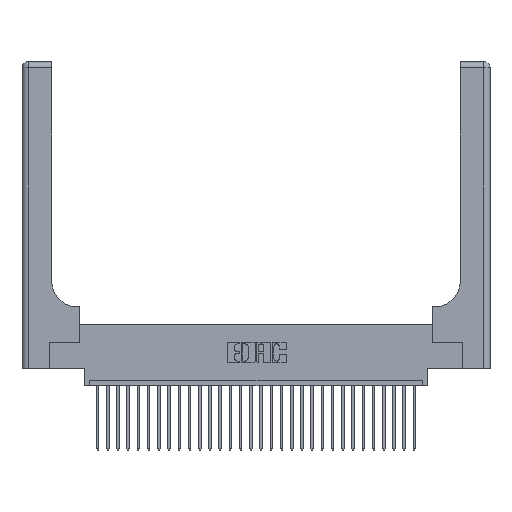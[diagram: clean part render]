
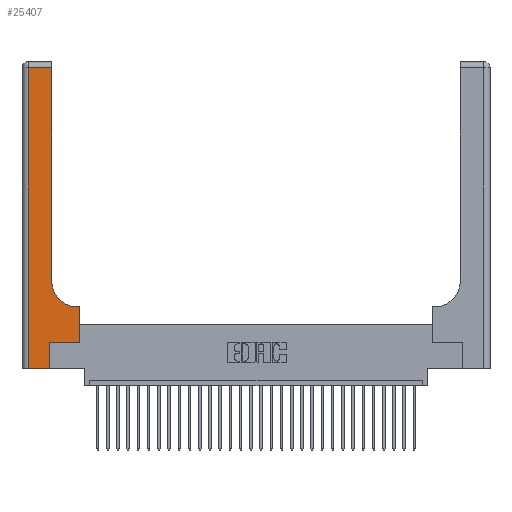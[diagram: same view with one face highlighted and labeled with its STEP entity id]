
A CAD part, top view. The second image highlights one B-rep face of the part: STEP entity #25407.
In plain terms, the highlighted planar face has unit normal (0, 0, 1).
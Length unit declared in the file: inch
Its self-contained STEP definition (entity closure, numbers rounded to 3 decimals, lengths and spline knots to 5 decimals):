
#1263 = CARTESIAN_POINT ( 'NONE',  ( 0.5415, 0.85, 0.37 ) ) ;
#1812 = FACE_OUTER_BOUND ( 'NONE', #27605, .T. ) ;
#2445 = CARTESIAN_POINT ( 'NONE',  ( 0.5415, 0.6, 0.37 ) ) ;
#2628 = EDGE_CURVE ( 'NONE', #19721, #12582, #14094, .T. ) ;
#2738 = CARTESIAN_POINT ( 'NONE',  ( 0.2915, 0.85, 0.37 ) ) ;
#2833 = VECTOR ( 'NONE', #13495, 39.37008 ) ;
#3415 = EDGE_CURVE ( 'NONE', #28434, #19721, #30053, .T. ) ;
#3424 = DIRECTION ( 'NONE',  ( 1., 0., 0. ) ) ;
#4033 = LINE ( 'NONE', #15360, #9617 ) ;
#4119 = EDGE_CURVE ( 'NONE', #24742, #16870, #18532, .T. ) ;
#4542 = VECTOR ( 'NONE', #12631, 39.37008 ) ;
#4820 = VECTOR ( 'NONE', #21781, 39.37008 ) ;
#4957 = LINE ( 'NONE', #10661, #13817 ) ;
#4981 = DIRECTION ( 'NONE',  ( 0., 0., -1. ) ) ;
#6355 = CARTESIAN_POINT ( 'NONE',  ( 0.5585, 0.25, 0.37 ) ) ;
#7140 = EDGE_CURVE ( 'NONE', #30685, #24742, #9123, .T. ) ;
#7196 = AXIS2_PLACEMENT_3D ( 'NONE', #23761, #4981, #26261 ) ;
#7293 = ORIENTED_EDGE ( 'NONE', *, *, #10783, .T. ) ;
#7933 = CARTESIAN_POINT ( 'NONE',  ( 0.5585, 0.25, 0.37 ) ) ;
#9074 = CARTESIAN_POINT ( 'NONE',  ( 0.269, 0.25, 0.37 ) ) ;
#9123 = LINE ( 'NONE', #6355, #10249 ) ;
#9617 = VECTOR ( 'NONE', #3424, 39.37008 ) ;
#10152 = ORIENTED_EDGE ( 'NONE', *, *, #29019, .T. ) ;
#10249 = VECTOR ( 'NONE', #18937, 39.37008 ) ;
#10362 = CARTESIAN_POINT ( 'NONE',  ( 0.2915, 3., 0.37 ) ) ;
#10658 = CIRCLE ( 'NONE', #14907, 0.25 ) ;
#10661 = CARTESIAN_POINT ( 'NONE',  ( 0., 2.94, 0.37 ) ) ;
#10696 = CARTESIAN_POINT ( 'NONE',  ( 0.06, 2.94, 0.37 ) ) ;
#10783 = EDGE_CURVE ( 'NONE', #23020, #30685, #4033, .T. ) ;
#10990 = DIRECTION ( 'NONE',  ( 0., 0., -1. ) ) ;
#11312 = ORIENTED_EDGE ( 'NONE', *, *, #7140, .T. ) ;
#11572 = DIRECTION ( 'NONE',  ( 1., 0., 0. ) ) ;
#12044 = EDGE_CURVE ( 'NONE', #16870, #23280, #10658, .T. ) ;
#12126 = ORIENTED_EDGE ( 'NONE', *, *, #29683, .T. ) ;
#12237 = PLANE ( 'NONE',  #7196 ) ;
#12582 = VERTEX_POINT ( 'NONE', #22857 ) ;
#12631 = DIRECTION ( 'NONE',  ( 0., 1., 0. ) ) ;
#12977 = ORIENTED_EDGE ( 'NONE', *, *, #2628, .T. ) ;
#13495 = DIRECTION ( 'NONE',  ( 0., 1., 0. ) ) ;
#13817 = VECTOR ( 'NONE', #27359, 39.37008 ) ;
#14094 = LINE ( 'NONE', #14251, #29005 ) ;
#14251 = CARTESIAN_POINT ( 'NONE',  ( 0., 0., 0.37 ) ) ;
#14380 = CARTESIAN_POINT ( 'NONE',  ( 0.06, 3., 0.37 ) ) ;
#14668 = CARTESIAN_POINT ( 'NONE',  ( 0.2915, 0.6, 0.37 ) ) ;
#14854 = ORIENTED_EDGE ( 'NONE', *, *, #12044, .T. ) ;
#14907 = AXIS2_PLACEMENT_3D ( 'NONE', #1263, #10990, #27188 ) ;
#15360 = CARTESIAN_POINT ( 'NONE',  ( 0.269, 0.25, 0.37 ) ) ;
#15441 = EDGE_CURVE ( 'NONE', #23280, #19581, #30542, .T. ) ;
#16237 = CARTESIAN_POINT ( 'NONE',  ( 0.269, 0., 0.37 ) ) ;
#16285 = VECTOR ( 'NONE', #19068, 39.37008 ) ;
#16870 = VERTEX_POINT ( 'NONE', #2445 ) ;
#17936 = ORIENTED_EDGE ( 'NONE', *, *, #4119, .T. ) ;
#18532 = LINE ( 'NONE', #14668, #16285 ) ;
#18937 = DIRECTION ( 'NONE',  ( 0., 1., 0. ) ) ;
#19068 = DIRECTION ( 'NONE',  ( -1., 0., 0. ) ) ;
#19570 = LINE ( 'NONE', #16237, #2833 ) ;
#19581 = VERTEX_POINT ( 'NONE', #28513 ) ;
#19721 = VERTEX_POINT ( 'NONE', #29220 ) ;
#21781 = DIRECTION ( 'NONE',  ( 0., -1., 0. ) ) ;
#22857 = CARTESIAN_POINT ( 'NONE',  ( 0.269, 0., 0.37 ) ) ;
#23020 = VERTEX_POINT ( 'NONE', #9074 ) ;
#23280 = VERTEX_POINT ( 'NONE', #2738 ) ;
#23761 = CARTESIAN_POINT ( 'NONE',  ( 0., 3., 0.37 ) ) ;
#24742 = VERTEX_POINT ( 'NONE', #28140 ) ;
#25407 = ADVANCED_FACE ( 'NONE', ( #1812 ), #12237, .F. ) ;
#26261 = DIRECTION ( 'NONE',  ( -1., 0., 0. ) ) ;
#27188 = DIRECTION ( 'NONE',  ( 1., 0., 0. ) ) ;
#27359 = DIRECTION ( 'NONE',  ( -1., 0., 0. ) ) ;
#27605 = EDGE_LOOP ( 'NONE', ( #28759, #10152, #29534, #12977, #12126, #7293, #11312, #17936, #14854 ) ) ;
#28140 = CARTESIAN_POINT ( 'NONE',  ( 0.5585, 0.6, 0.37 ) ) ;
#28434 = VERTEX_POINT ( 'NONE', #10696 ) ;
#28513 = CARTESIAN_POINT ( 'NONE',  ( 0.2915, 2.94, 0.37 ) ) ;
#28759 = ORIENTED_EDGE ( 'NONE', *, *, #15441, .T. ) ;
#29005 = VECTOR ( 'NONE', #11572, 39.37008 ) ;
#29019 = EDGE_CURVE ( 'NONE', #19581, #28434, #4957, .T. ) ;
#29220 = CARTESIAN_POINT ( 'NONE',  ( 0.06, 0., 0.37 ) ) ;
#29534 = ORIENTED_EDGE ( 'NONE', *, *, #3415, .T. ) ;
#29683 = EDGE_CURVE ( 'NONE', #12582, #23020, #19570, .T. ) ;
#30053 = LINE ( 'NONE', #14380, #4820 ) ;
#30542 = LINE ( 'NONE', #10362, #4542 ) ;
#30685 = VERTEX_POINT ( 'NONE', #7933 ) ;
